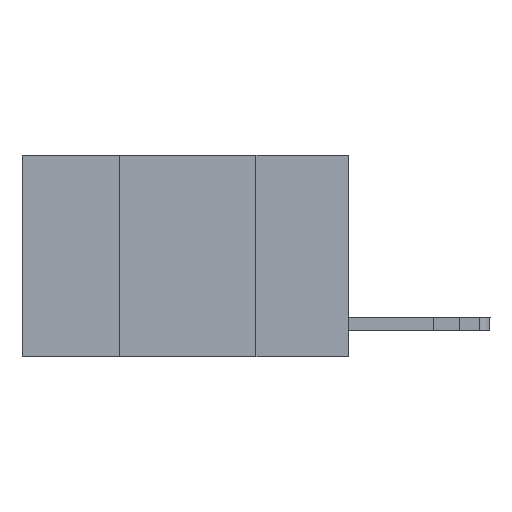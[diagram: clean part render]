
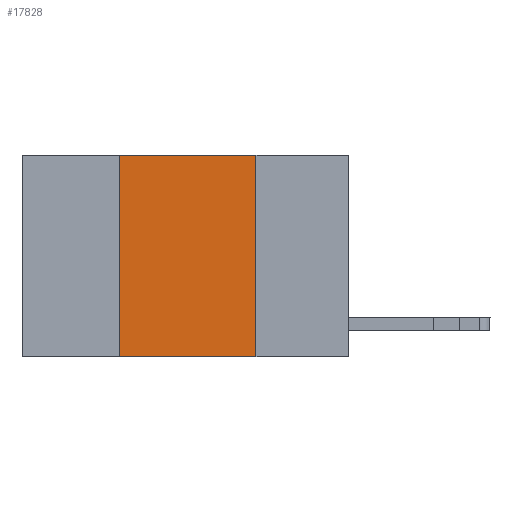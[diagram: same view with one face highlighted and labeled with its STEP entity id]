
A CAD part, left-side view. The second image highlights one B-rep face of the part: STEP entity #17828.
In plain terms, the highlighted planar face has unit normal (-1, 0, 0).
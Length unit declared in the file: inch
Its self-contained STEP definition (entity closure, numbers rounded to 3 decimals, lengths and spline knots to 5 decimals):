
#261 = ORIENTED_EDGE ( 'NONE', *, *, #4533, .F. ) ;
#493 = ORIENTED_EDGE ( 'NONE', *, *, #5024, .F. ) ;
#662 = VECTOR ( 'NONE', #1603, 39.37008 ) ;
#1603 = DIRECTION ( 'NONE',  ( 0., -1., 0. ) ) ;
#2409 = EDGE_LOOP ( 'NONE', ( #19608, #493, #261, #19333 ) ) ;
#3246 = CARTESIAN_POINT ( 'NONE',  ( 0., 0.6, 0. ) ) ;
#3772 = CARTESIAN_POINT ( 'NONE',  ( 0., 0.42, 0. ) ) ;
#4212 = CARTESIAN_POINT ( 'NONE',  ( 0., 0.17, 0. ) ) ;
#4533 = EDGE_CURVE ( 'NONE', #11600, #10154, #20541, .T. ) ;
#5024 = EDGE_CURVE ( 'NONE', #10154, #9303, #5158, .T. ) ;
#5158 = LINE ( 'NONE', #3246, #662 ) ;
#5198 = DIRECTION ( 'NONE',  ( 0., -1., 0. ) ) ;
#6369 = VECTOR ( 'NONE', #10515, 39.37008 ) ;
#7625 = CARTESIAN_POINT ( 'NONE',  ( 0., 0.6, 0. ) ) ;
#8403 = CARTESIAN_POINT ( 'NONE',  ( 0., 0.42, 0. ) ) ;
#9287 = DIRECTION ( 'NONE',  ( 0., 0., -1. ) ) ;
#9303 = VERTEX_POINT ( 'NONE', #4212 ) ;
#10154 = VERTEX_POINT ( 'NONE', #8403 ) ;
#10515 = DIRECTION ( 'NONE',  ( 0., 0., -1. ) ) ;
#10879 = PLANE ( 'NONE',  #20882 ) ;
#10920 = VECTOR ( 'NONE', #5198, 39.37008 ) ;
#11288 = VECTOR ( 'NONE', #13707, 39.37008 ) ;
#11412 = FACE_OUTER_BOUND ( 'NONE', #2409, .T. ) ;
#11600 = VERTEX_POINT ( 'NONE', #18735 ) ;
#11809 = CARTESIAN_POINT ( 'NONE',  ( 0., 0.6, -0.37 ) ) ;
#12224 = CARTESIAN_POINT ( 'NONE',  ( 0., 0.17, 0. ) ) ;
#12918 = EDGE_CURVE ( 'NONE', #11600, #14188, #16315, .T. ) ;
#13707 = DIRECTION ( 'NONE',  ( 0., 0., 1. ) ) ;
#14188 = VERTEX_POINT ( 'NONE', #18307 ) ;
#15135 = LINE ( 'NONE', #12224, #6369 ) ;
#16315 = LINE ( 'NONE', #11809, #10920 ) ;
#17828 = ADVANCED_FACE ( 'NONE', ( #11412 ), #10879, .F. ) ;
#18307 = CARTESIAN_POINT ( 'NONE',  ( 0., 0.17, -0.37 ) ) ;
#18735 = CARTESIAN_POINT ( 'NONE',  ( 0., 0.42, -0.37 ) ) ;
#19156 = DIRECTION ( 'NONE',  ( 1., 0., 0. ) ) ;
#19333 = ORIENTED_EDGE ( 'NONE', *, *, #12918, .T. ) ;
#19608 = ORIENTED_EDGE ( 'NONE', *, *, #20913, .F. ) ;
#20541 = LINE ( 'NONE', #3772, #11288 ) ;
#20882 = AXIS2_PLACEMENT_3D ( 'NONE', #7625, #19156, #9287 ) ;
#20913 = EDGE_CURVE ( 'NONE', #9303, #14188, #15135, .T. ) ;
